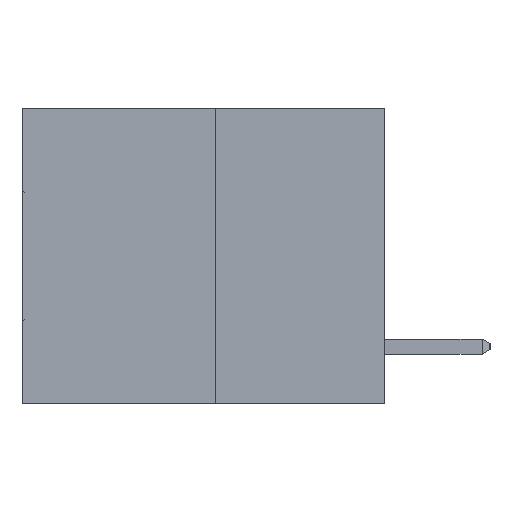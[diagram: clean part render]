
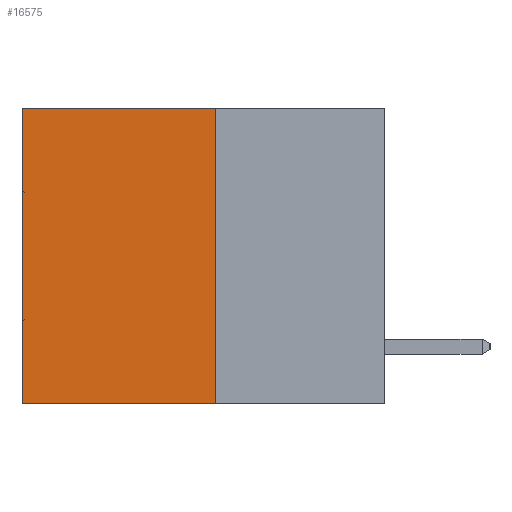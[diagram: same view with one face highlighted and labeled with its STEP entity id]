
A CAD part, left-side view. The second image highlights one B-rep face of the part: STEP entity #16575.
In plain terms, the highlighted planar face has unit normal (-1, 0, 0).
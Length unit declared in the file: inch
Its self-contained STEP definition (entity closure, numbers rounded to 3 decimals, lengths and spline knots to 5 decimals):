
#1503 = VECTOR ( 'NONE', #21220, 39.37008 ) ;
#2016 = FACE_OUTER_BOUND ( 'NONE', #17096, .T. ) ;
#2089 = CARTESIAN_POINT ( 'NONE',  ( 0.3165, 0.28, 0. ) ) ;
#2274 = DIRECTION ( 'NONE',  ( 0., 0., -1. ) ) ;
#4056 = VECTOR ( 'NONE', #9771, 39.37008 ) ;
#5459 = VECTOR ( 'NONE', #29303, 39.37008 ) ;
#6826 = EDGE_CURVE ( 'NONE', #17948, #23525, #24983, .T. ) ;
#7454 = PLANE ( 'NONE',  #28040 ) ;
#8387 = VERTEX_POINT ( 'NONE', #19519 ) ;
#9454 = LINE ( 'NONE', #2089, #1503 ) ;
#9771 = DIRECTION ( 'NONE',  ( 0., 1., 0. ) ) ;
#9818 = CARTESIAN_POINT ( 'NONE',  ( 0.3165, 0.6, -0.49 ) ) ;
#16255 = EDGE_CURVE ( 'NONE', #8387, #23525, #19557, .T. ) ;
#16575 = ADVANCED_FACE ( 'NONE', ( #2016 ), #7454, .F. ) ;
#16584 = ORIENTED_EDGE ( 'NONE', *, *, #6826, .F. ) ;
#16594 = LINE ( 'NONE', #16657, #19624 ) ;
#16657 = CARTESIAN_POINT ( 'NONE',  ( 0.3165, 0.28, -0.49 ) ) ;
#16863 = DIRECTION ( 'NONE',  ( 1., 0., 0. ) ) ;
#17096 = EDGE_LOOP ( 'NONE', ( #23701, #16584, #24952, #28735 ) ) ;
#17948 = VERTEX_POINT ( 'NONE', #21923 ) ;
#18916 = EDGE_CURVE ( 'NONE', #28778, #8387, #9454, .T. ) ;
#19519 = CARTESIAN_POINT ( 'NONE',  ( 0.3165, 0.6, 0. ) ) ;
#19557 = LINE ( 'NONE', #9818, #5459 ) ;
#19624 = VECTOR ( 'NONE', #26415, 39.37008 ) ;
#21220 = DIRECTION ( 'NONE',  ( 0., 1., 0. ) ) ;
#21876 = CARTESIAN_POINT ( 'NONE',  ( 0.3165, 0.6, -0.49 ) ) ;
#21923 = CARTESIAN_POINT ( 'NONE',  ( 0.3165, 0.28, -0.49 ) ) ;
#23525 = VERTEX_POINT ( 'NONE', #21876 ) ;
#23701 = ORIENTED_EDGE ( 'NONE', *, *, #16255, .T. ) ;
#23967 = CARTESIAN_POINT ( 'NONE',  ( 0.3165, 0.28, -0.49 ) ) ;
#24952 = ORIENTED_EDGE ( 'NONE', *, *, #30644, .F. ) ;
#24983 = LINE ( 'NONE', #23967, #4056 ) ;
#26415 = DIRECTION ( 'NONE',  ( 0., 0., -1. ) ) ;
#28040 = AXIS2_PLACEMENT_3D ( 'NONE', #29166, #16863, #2274 ) ;
#28136 = CARTESIAN_POINT ( 'NONE',  ( 0.3165, 0.28, 0. ) ) ;
#28735 = ORIENTED_EDGE ( 'NONE', *, *, #18916, .T. ) ;
#28778 = VERTEX_POINT ( 'NONE', #28136 ) ;
#29166 = CARTESIAN_POINT ( 'NONE',  ( 0.3165, 0.28, -0.49 ) ) ;
#29303 = DIRECTION ( 'NONE',  ( 0., 0., -1. ) ) ;
#30644 = EDGE_CURVE ( 'NONE', #28778, #17948, #16594, .T. ) ;
